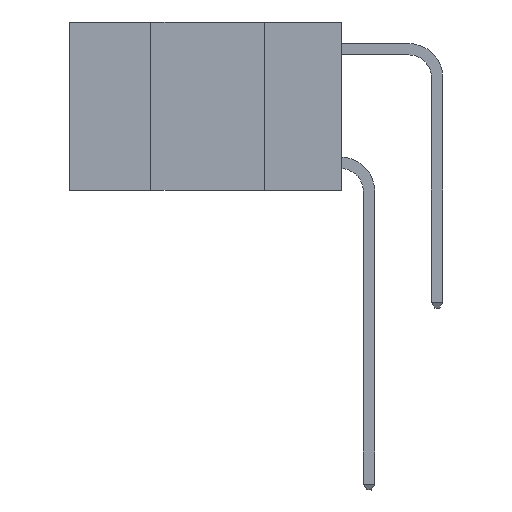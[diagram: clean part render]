
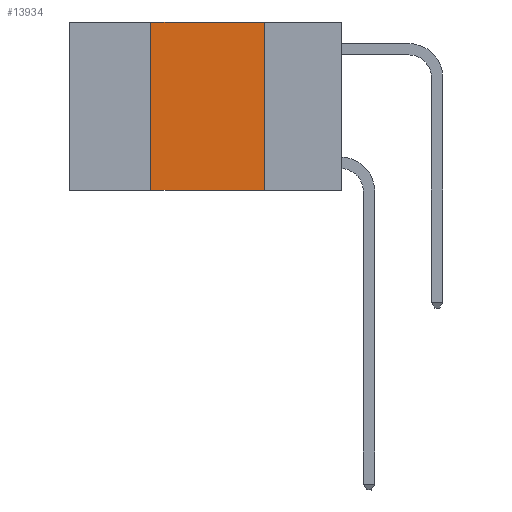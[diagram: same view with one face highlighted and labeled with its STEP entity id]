
A CAD part, left-side view. The second image highlights one B-rep face of the part: STEP entity #13934.
In plain terms, the highlighted planar face has unit normal (-1, 0, 0).
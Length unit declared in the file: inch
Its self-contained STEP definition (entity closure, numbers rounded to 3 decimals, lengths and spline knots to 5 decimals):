
#257 = DIRECTION ( 'NONE',  ( 0., 0., -1. ) ) ;
#699 = CARTESIAN_POINT ( 'NONE',  ( 0., 0.42, 0. ) ) ;
#899 = CARTESIAN_POINT ( 'NONE',  ( 0., 0.17, -0.37 ) ) ;
#1587 = VECTOR ( 'NONE', #11791, 39.37008 ) ;
#1700 = LINE ( 'NONE', #5338, #2688 ) ;
#1778 = DIRECTION ( 'NONE',  ( 0., -1., 0. ) ) ;
#2688 = VECTOR ( 'NONE', #1778, 39.37008 ) ;
#2929 = VERTEX_POINT ( 'NONE', #9312 ) ;
#3443 = EDGE_CURVE ( 'NONE', #2929, #13684, #8556, .T. ) ;
#3899 = AXIS2_PLACEMENT_3D ( 'NONE', #11202, #5153, #257 ) ;
#4353 = ORIENTED_EDGE ( 'NONE', *, *, #13436, .F. ) ;
#4793 = CARTESIAN_POINT ( 'NONE',  ( 0., 0.17, 0. ) ) ;
#4910 = EDGE_CURVE ( 'NONE', #7669, #13684, #1700, .T. ) ;
#5153 = DIRECTION ( 'NONE',  ( 1., 0., 0. ) ) ;
#5230 = PLANE ( 'NONE',  #3899 ) ;
#5333 = CARTESIAN_POINT ( 'NONE',  ( 0., 0.42, 0. ) ) ;
#5338 = CARTESIAN_POINT ( 'NONE',  ( 0., 0.6, -0.37 ) ) ;
#7502 = LINE ( 'NONE', #5333, #11373 ) ;
#7669 = VERTEX_POINT ( 'NONE', #12045 ) ;
#8556 = LINE ( 'NONE', #4793, #8884 ) ;
#8884 = VECTOR ( 'NONE', #12174, 39.37008 ) ;
#9102 = EDGE_CURVE ( 'NONE', #9232, #2929, #9154, .T. ) ;
#9154 = LINE ( 'NONE', #11487, #1587 ) ;
#9232 = VERTEX_POINT ( 'NONE', #699 ) ;
#9312 = CARTESIAN_POINT ( 'NONE',  ( 0., 0.17, 0. ) ) ;
#10255 = ORIENTED_EDGE ( 'NONE', *, *, #3443, .F. ) ;
#10342 = ORIENTED_EDGE ( 'NONE', *, *, #9102, .F. ) ;
#11202 = CARTESIAN_POINT ( 'NONE',  ( 0., 0.6, 0. ) ) ;
#11373 = VECTOR ( 'NONE', #13835, 39.37008 ) ;
#11487 = CARTESIAN_POINT ( 'NONE',  ( 0., 0.6, 0. ) ) ;
#11791 = DIRECTION ( 'NONE',  ( 0., -1., 0. ) ) ;
#12045 = CARTESIAN_POINT ( 'NONE',  ( 0., 0.42, -0.37 ) ) ;
#12174 = DIRECTION ( 'NONE',  ( 0., 0., -1. ) ) ;
#13436 = EDGE_CURVE ( 'NONE', #7669, #9232, #7502, .T. ) ;
#13684 = VERTEX_POINT ( 'NONE', #899 ) ;
#13835 = DIRECTION ( 'NONE',  ( 0., 0., 1. ) ) ;
#13934 = ADVANCED_FACE ( 'NONE', ( #14871 ), #5230, .F. ) ;
#14582 = EDGE_LOOP ( 'NONE', ( #10255, #10342, #4353, #15735 ) ) ;
#14871 = FACE_OUTER_BOUND ( 'NONE', #14582, .T. ) ;
#15735 = ORIENTED_EDGE ( 'NONE', *, *, #4910, .T. ) ;
